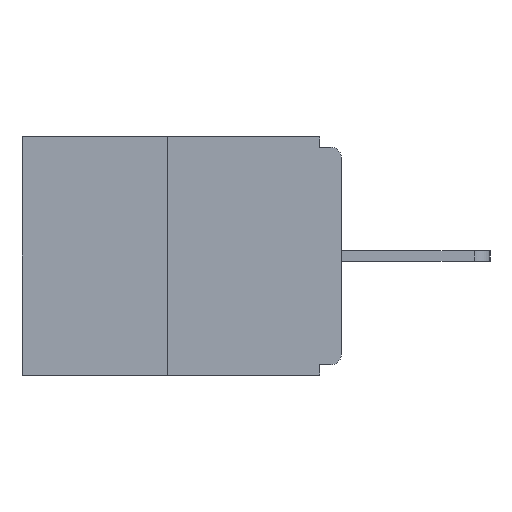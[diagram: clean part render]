
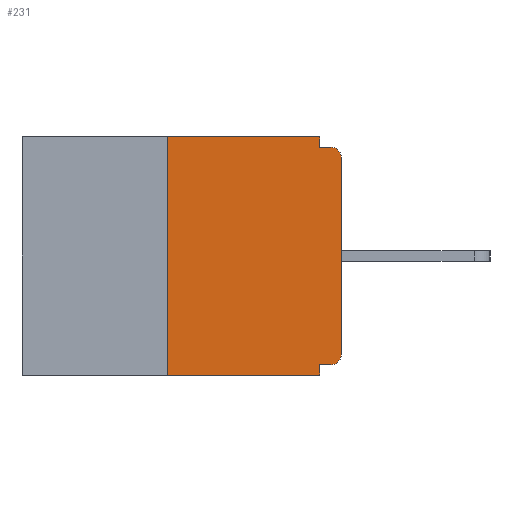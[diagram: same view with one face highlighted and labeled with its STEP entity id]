
A CAD part, left-side view. The second image highlights one B-rep face of the part: STEP entity #231.
In plain terms, the highlighted planar face has unit normal (-1, 0, 0).
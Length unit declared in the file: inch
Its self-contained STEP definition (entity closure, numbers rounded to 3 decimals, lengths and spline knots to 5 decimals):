
#70 = EDGE_CURVE ( 'NONE', #7647, #9649, #2889, .T. ) ;
#231 = ADVANCED_FACE ( 'NONE', ( #8801 ), #3535, .F. ) ;
#238 = DIRECTION ( 'NONE',  ( 0., -1., 0. ) ) ;
#461 = VERTEX_POINT ( 'NONE', #7467 ) ;
#761 = VERTEX_POINT ( 'NONE', #10868 ) ;
#1019 = VECTOR ( 'NONE', #10810, 39.37008 ) ;
#1042 = CARTESIAN_POINT ( 'NONE',  ( 0., 0.46, -0.343 ) ) ;
#1089 = EDGE_CURVE ( 'NONE', #6716, #3776, #11395, .T. ) ;
#1170 = CIRCLE ( 'NONE', #2716, 0.015 ) ;
#1199 = CARTESIAN_POINT ( 'NONE',  ( 0., 0.015, -0.03 ) ) ;
#1381 = CARTESIAN_POINT ( 'NONE',  ( 0., 0.031, 0. ) ) ;
#1477 = ORIENTED_EDGE ( 'NONE', *, *, #1089, .F. ) ;
#1516 = ORIENTED_EDGE ( 'NONE', *, *, #1764, .T. ) ;
#1764 = EDGE_CURVE ( 'NONE', #10398, #2778, #9563, .T. ) ;
#1779 = CARTESIAN_POINT ( 'NONE',  ( 0., 0.031, -0.343 ) ) ;
#2024 = DIRECTION ( 'NONE',  ( 0., 0., -1. ) ) ;
#2568 = EDGE_CURVE ( 'NONE', #4107, #3045, #3232, .T. ) ;
#2709 = CARTESIAN_POINT ( 'NONE',  ( 0., 0.015, -0.313 ) ) ;
#2716 = AXIS2_PLACEMENT_3D ( 'NONE', #1199, #7595, #9631 ) ;
#2736 = LINE ( 'NONE', #6324, #8515 ) ;
#2778 = VERTEX_POINT ( 'NONE', #10099 ) ;
#2889 = LINE ( 'NONE', #3660, #3236 ) ;
#2964 = LINE ( 'NONE', #10093, #7038 ) ;
#2990 = CARTESIAN_POINT ( 'NONE',  ( 0., 0., -0.015 ) ) ;
#3045 = VERTEX_POINT ( 'NONE', #6311 ) ;
#3232 = LINE ( 'NONE', #2990, #10891 ) ;
#3236 = VECTOR ( 'NONE', #4679, 39.37008 ) ;
#3466 = ORIENTED_EDGE ( 'NONE', *, *, #2568, .F. ) ;
#3535 = PLANE ( 'NONE',  #8198 ) ;
#3660 = CARTESIAN_POINT ( 'NONE',  ( 0., 0.031, -0.343 ) ) ;
#3772 = EDGE_CURVE ( 'NONE', #761, #3045, #1170, .T. ) ;
#3776 = VERTEX_POINT ( 'NONE', #1381 ) ;
#3993 = EDGE_LOOP ( 'NONE', ( #1477, #10124, #10283, #9118, #8148, #1516, #10468, #9654, #3466, #9798 ) ) ;
#4043 = CARTESIAN_POINT ( 'NONE',  ( 0., 0.015, -0.328 ) ) ;
#4091 = VECTOR ( 'NONE', #4700, 39.37008 ) ;
#4107 = VERTEX_POINT ( 'NONE', #6398 ) ;
#4230 = LINE ( 'NONE', #11539, #1019 ) ;
#4589 = CARTESIAN_POINT ( 'NONE',  ( 0., 0.25, 0. ) ) ;
#4675 = CARTESIAN_POINT ( 'NONE',  ( 0., 0.031, -0.328 ) ) ;
#4679 = DIRECTION ( 'NONE',  ( 0., 0., -1. ) ) ;
#4700 = DIRECTION ( 'NONE',  ( 0., -1., 0. ) ) ;
#5000 = DIRECTION ( 'NONE',  ( 0., 0., -1. ) ) ;
#5164 = LINE ( 'NONE', #8797, #6098 ) ;
#5266 = EDGE_CURVE ( 'NONE', #10398, #7647, #5164, .T. ) ;
#5434 = DIRECTION ( 'NONE',  ( 0., 0., 1. ) ) ;
#5596 = LINE ( 'NONE', #1042, #4091 ) ;
#5829 = CARTESIAN_POINT ( 'NONE',  ( 0., 0.46, 0. ) ) ;
#6074 = EDGE_CURVE ( 'NONE', #461, #6716, #4230, .T. ) ;
#6098 = VECTOR ( 'NONE', #7900, 39.37008 ) ;
#6311 = CARTESIAN_POINT ( 'NONE',  ( 0., 0.015, -0.015 ) ) ;
#6324 = CARTESIAN_POINT ( 'NONE',  ( 0., 0., 0. ) ) ;
#6398 = CARTESIAN_POINT ( 'NONE',  ( 0., 0.031, -0.015 ) ) ;
#6461 = DIRECTION ( 'NONE',  ( -1., 0., 0. ) ) ;
#6716 = VERTEX_POINT ( 'NONE', #4589 ) ;
#6940 = DIRECTION ( 'NONE',  ( 0., 0., -1. ) ) ;
#6961 = EDGE_CURVE ( 'NONE', #461, #9649, #5596, .T. ) ;
#7038 = VECTOR ( 'NONE', #5000, 39.37008 ) ;
#7467 = CARTESIAN_POINT ( 'NONE',  ( 0., 0.25, -0.343 ) ) ;
#7595 = DIRECTION ( 'NONE',  ( -1., 0., 0. ) ) ;
#7647 = VERTEX_POINT ( 'NONE', #4675 ) ;
#7900 = DIRECTION ( 'NONE',  ( 0., 1., 0. ) ) ;
#8036 = AXIS2_PLACEMENT_3D ( 'NONE', #2709, #6461, #2024 ) ;
#8148 = ORIENTED_EDGE ( 'NONE', *, *, #5266, .F. ) ;
#8198 = AXIS2_PLACEMENT_3D ( 'NONE', #11631, #11510, #6940 ) ;
#8515 = VECTOR ( 'NONE', #5434, 39.37008 ) ;
#8797 = CARTESIAN_POINT ( 'NONE',  ( 0., 0., -0.328 ) ) ;
#8801 = FACE_OUTER_BOUND ( 'NONE', #3993, .T. ) ;
#9118 = ORIENTED_EDGE ( 'NONE', *, *, #70, .F. ) ;
#9474 = DIRECTION ( 'NONE',  ( 0., -1., 0. ) ) ;
#9563 = CIRCLE ( 'NONE', #8036, 0.015 ) ;
#9631 = DIRECTION ( 'NONE',  ( 0., 0., -1. ) ) ;
#9649 = VERTEX_POINT ( 'NONE', #1779 ) ;
#9654 = ORIENTED_EDGE ( 'NONE', *, *, #3772, .T. ) ;
#9783 = EDGE_CURVE ( 'NONE', #3776, #4107, #2964, .T. ) ;
#9798 = ORIENTED_EDGE ( 'NONE', *, *, #9783, .F. ) ;
#10093 = CARTESIAN_POINT ( 'NONE',  ( 0., 0.031, 0. ) ) ;
#10099 = CARTESIAN_POINT ( 'NONE',  ( 0., 0., -0.313 ) ) ;
#10124 = ORIENTED_EDGE ( 'NONE', *, *, #6074, .F. ) ;
#10187 = VECTOR ( 'NONE', #9474, 39.37008 ) ;
#10283 = ORIENTED_EDGE ( 'NONE', *, *, #6961, .T. ) ;
#10398 = VERTEX_POINT ( 'NONE', #4043 ) ;
#10468 = ORIENTED_EDGE ( 'NONE', *, *, #11546, .T. ) ;
#10810 = DIRECTION ( 'NONE',  ( 0., 0., 1. ) ) ;
#10868 = CARTESIAN_POINT ( 'NONE',  ( 0., 0., -0.03 ) ) ;
#10891 = VECTOR ( 'NONE', #238, 39.37008 ) ;
#11395 = LINE ( 'NONE', #5829, #10187 ) ;
#11510 = DIRECTION ( 'NONE',  ( 1., 0., 0. ) ) ;
#11539 = CARTESIAN_POINT ( 'NONE',  ( 0., 0.25, 0. ) ) ;
#11546 = EDGE_CURVE ( 'NONE', #2778, #761, #2736, .T. ) ;
#11631 = CARTESIAN_POINT ( 'NONE',  ( 0., 0.46, 0. ) ) ;
